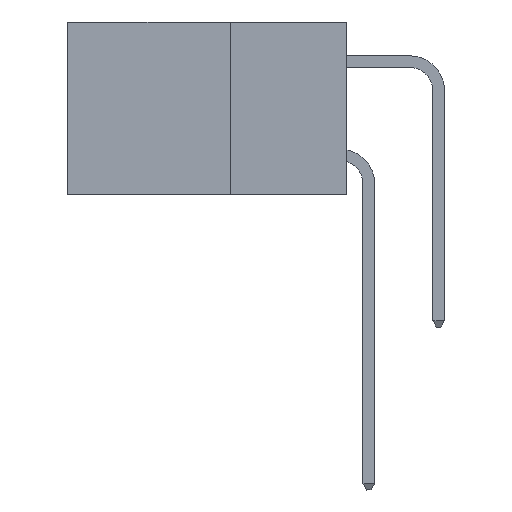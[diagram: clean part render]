
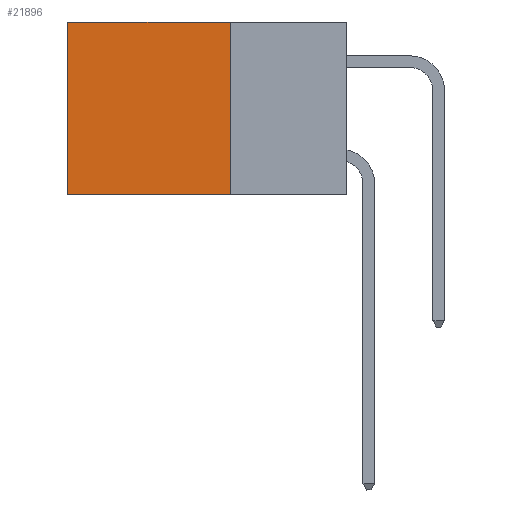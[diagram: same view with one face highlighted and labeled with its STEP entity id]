
A CAD part, left-side view. The second image highlights one B-rep face of the part: STEP entity #21896.
In plain terms, the highlighted planar face has unit normal (-1, 0, 0).
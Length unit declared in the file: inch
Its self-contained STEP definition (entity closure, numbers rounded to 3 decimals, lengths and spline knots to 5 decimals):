
#140 = DIRECTION ( 'NONE',  ( 1., 0., 0. ) ) ;
#204 = CARTESIAN_POINT ( 'NONE',  ( 0.2875, 0.6, 0. ) ) ;
#221 = VECTOR ( 'NONE', #13783, 39.37008 ) ;
#1746 = ORIENTED_EDGE ( 'NONE', *, *, #10603, .T. ) ;
#2792 = CARTESIAN_POINT ( 'NONE',  ( 0.2875, 0.25, 0. ) ) ;
#2983 = LINE ( 'NONE', #25949, #9122 ) ;
#3996 = VERTEX_POINT ( 'NONE', #26658 ) ;
#4393 = EDGE_LOOP ( 'NONE', ( #20339, #15331, #35946, #1746 ) ) ;
#4405 = CARTESIAN_POINT ( 'NONE',  ( 0.2875, 0.25, -0.37 ) ) ;
#5247 = VERTEX_POINT ( 'NONE', #32247 ) ;
#5967 = FACE_OUTER_BOUND ( 'NONE', #4393, .T. ) ;
#7305 = CARTESIAN_POINT ( 'NONE',  ( 0.2875, 0.6, 0. ) ) ;
#7711 = LINE ( 'NONE', #7305, #22788 ) ;
#9122 = VECTOR ( 'NONE', #16961, 39.37008 ) ;
#10364 = CARTESIAN_POINT ( 'NONE',  ( 0.2875, 0.25, 0. ) ) ;
#10603 = EDGE_CURVE ( 'NONE', #3996, #23807, #2983, .T. ) ;
#11107 = LINE ( 'NONE', #10364, #21951 ) ;
#11998 = DIRECTION ( 'NONE',  ( 0., 0., -1. ) ) ;
#13783 = DIRECTION ( 'NONE',  ( 0., 1., 0. ) ) ;
#15331 = ORIENTED_EDGE ( 'NONE', *, *, #36360, .F. ) ;
#16400 = DIRECTION ( 'NONE',  ( 0., 0., -1. ) ) ;
#16961 = DIRECTION ( 'NONE',  ( 0., 1., 0. ) ) ;
#19292 = DIRECTION ( 'NONE',  ( 0., 0., -1. ) ) ;
#20312 = VERTEX_POINT ( 'NONE', #31506 ) ;
#20339 = ORIENTED_EDGE ( 'NONE', *, *, #23979, .T. ) ;
#21896 = ADVANCED_FACE ( 'NONE', ( #5967 ), #38933, .F. ) ;
#21951 = VECTOR ( 'NONE', #16400, 39.37008 ) ;
#22147 = EDGE_CURVE ( 'NONE', #3996, #5247, #11107, .T. ) ;
#22788 = VECTOR ( 'NONE', #19292, 39.37008 ) ;
#23807 = VERTEX_POINT ( 'NONE', #204 ) ;
#23957 = AXIS2_PLACEMENT_3D ( 'NONE', #2792, #140, #11998 ) ;
#23979 = EDGE_CURVE ( 'NONE', #23807, #20312, #7711, .T. ) ;
#25949 = CARTESIAN_POINT ( 'NONE',  ( 0.2875, 0.25, 0. ) ) ;
#26658 = CARTESIAN_POINT ( 'NONE',  ( 0.2875, 0.25, 0. ) ) ;
#29957 = LINE ( 'NONE', #4405, #221 ) ;
#31506 = CARTESIAN_POINT ( 'NONE',  ( 0.2875, 0.6, -0.37 ) ) ;
#32247 = CARTESIAN_POINT ( 'NONE',  ( 0.2875, 0.25, -0.37 ) ) ;
#35946 = ORIENTED_EDGE ( 'NONE', *, *, #22147, .F. ) ;
#36360 = EDGE_CURVE ( 'NONE', #5247, #20312, #29957, .T. ) ;
#38933 = PLANE ( 'NONE',  #23957 ) ;
